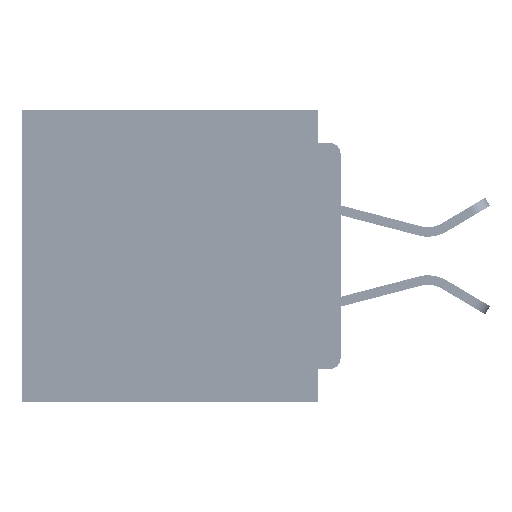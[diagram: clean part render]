
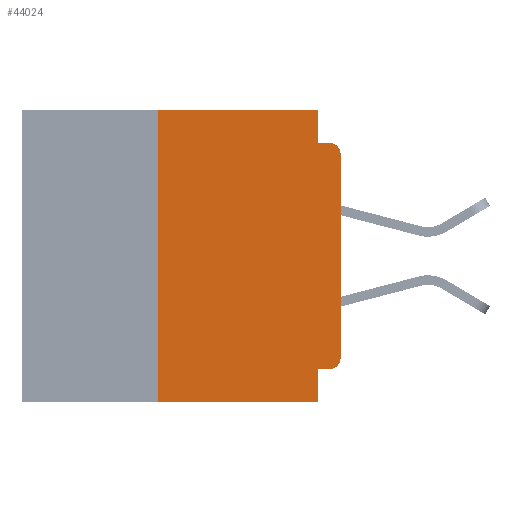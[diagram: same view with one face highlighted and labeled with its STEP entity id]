
A CAD part, left-side view. The second image highlights one B-rep face of the part: STEP entity #44024.
In plain terms, the highlighted planar face has unit normal (-1, 0, 0).
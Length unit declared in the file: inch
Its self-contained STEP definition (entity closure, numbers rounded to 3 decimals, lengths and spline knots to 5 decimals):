
#98 = DIRECTION ( 'NONE',  ( 1., 0., 0. ) ) ;
#563 = CARTESIAN_POINT ( 'NONE',  ( 0., 0.437, 0. ) ) ;
#869 = CIRCLE ( 'NONE', #25899, 0.015 ) ;
#2628 = VERTEX_POINT ( 'NONE', #38339 ) ;
#2960 = DIRECTION ( 'NONE',  ( -1., 0., 0. ) ) ;
#3124 = CIRCLE ( 'NONE', #36083, 0.015 ) ;
#3343 = EDGE_LOOP ( 'NONE', ( #52701, #41133, #58775, #60314, #26723, #52760, #15186, #45871, #8258, #12189 ) ) ;
#4657 = VERTEX_POINT ( 'NONE', #30805 ) ;
#6413 = VECTOR ( 'NONE', #18848, 39.37008 ) ;
#7046 = CARTESIAN_POINT ( 'NONE',  ( 0., 0.031, 0. ) ) ;
#7958 = LINE ( 'NONE', #43260, #6413 ) ;
#8258 = ORIENTED_EDGE ( 'NONE', *, *, #57988, .F. ) ;
#8402 = DIRECTION ( 'NONE',  ( 0., 1., 0. ) ) ;
#9303 = VERTEX_POINT ( 'NONE', #39330 ) ;
#12189 = ORIENTED_EDGE ( 'NONE', *, *, #32859, .T. ) ;
#14083 = LINE ( 'NONE', #53058, #51657 ) ;
#15186 = ORIENTED_EDGE ( 'NONE', *, *, #61107, .T. ) ;
#17028 = LINE ( 'NONE', #18074, #39983 ) ;
#18074 = CARTESIAN_POINT ( 'NONE',  ( 0., 0., -0.355 ) ) ;
#18848 = DIRECTION ( 'NONE',  ( 0., 0., -1. ) ) ;
#20015 = CARTESIAN_POINT ( 'NONE',  ( 0., 0.015, -0.355 ) ) ;
#20084 = CARTESIAN_POINT ( 'NONE',  ( 0., 0.437, -0.4 ) ) ;
#20939 = CARTESIAN_POINT ( 'NONE',  ( 0., 0.25, -0.4 ) ) ;
#21856 = LINE ( 'NONE', #30846, #47942 ) ;
#22065 = EDGE_CURVE ( 'NONE', #60674, #9303, #14083, .T. ) ;
#22498 = DIRECTION ( 'NONE',  ( 0., -1., 0. ) ) ;
#23489 = EDGE_CURVE ( 'NONE', #28039, #43343, #21856, .T. ) ;
#23637 = LINE ( 'NONE', #20084, #48149 ) ;
#24789 = CARTESIAN_POINT ( 'NONE',  ( 0., 0., -0.06 ) ) ;
#25058 = DIRECTION ( 'NONE',  ( 0., -1., 0. ) ) ;
#25899 = AXIS2_PLACEMENT_3D ( 'NONE', #56039, #26727, #60895 ) ;
#26045 = VECTOR ( 'NONE', #35021, 39.37008 ) ;
#26723 = ORIENTED_EDGE ( 'NONE', *, *, #46386, .F. ) ;
#26727 = DIRECTION ( 'NONE',  ( -1., 0., 0. ) ) ;
#28039 = VERTEX_POINT ( 'NONE', #62987 ) ;
#28452 = DIRECTION ( 'NONE',  ( 0., 0., -1. ) ) ;
#29638 = PLANE ( 'NONE',  #37920 ) ;
#30805 = CARTESIAN_POINT ( 'NONE',  ( 0., 0.015, -0.045 ) ) ;
#30846 = CARTESIAN_POINT ( 'NONE',  ( 0., 0., 0. ) ) ;
#31101 = CARTESIAN_POINT ( 'NONE',  ( 0., 0.25, -0.4 ) ) ;
#32452 = CARTESIAN_POINT ( 'NONE',  ( 0., 0.015, -0.34 ) ) ;
#32859 = EDGE_CURVE ( 'NONE', #36303, #28039, #3124, .T. ) ;
#34471 = CARTESIAN_POINT ( 'NONE',  ( 0., 0.031, -0.4 ) ) ;
#34568 = DIRECTION ( 'NONE',  ( 0., 0., -1. ) ) ;
#35021 = DIRECTION ( 'NONE',  ( 0., -1., 0. ) ) ;
#35789 = EDGE_CURVE ( 'NONE', #41170, #2628, #40969, .T. ) ;
#35803 = VECTOR ( 'NONE', #22498, 39.37008 ) ;
#36083 = AXIS2_PLACEMENT_3D ( 'NONE', #32452, #2960, #37370 ) ;
#36303 = VERTEX_POINT ( 'NONE', #20015 ) ;
#37370 = DIRECTION ( 'NONE',  ( 0., 0., -1. ) ) ;
#37485 = LINE ( 'NONE', #563, #26045 ) ;
#37920 = AXIS2_PLACEMENT_3D ( 'NONE', #44146, #98, #34568 ) ;
#38339 = CARTESIAN_POINT ( 'NONE',  ( 0., 0.25, 0. ) ) ;
#38690 = VERTEX_POINT ( 'NONE', #41377 ) ;
#38811 = LINE ( 'NONE', #61409, #35803 ) ;
#39330 = CARTESIAN_POINT ( 'NONE',  ( 0., 0.031, -0.045 ) ) ;
#39983 = VECTOR ( 'NONE', #8402, 39.37008 ) ;
#40969 = LINE ( 'NONE', #20939, #52534 ) ;
#41133 = ORIENTED_EDGE ( 'NONE', *, *, #48508, .T. ) ;
#41170 = VERTEX_POINT ( 'NONE', #31101 ) ;
#41377 = CARTESIAN_POINT ( 'NONE',  ( 0., 0.031, -0.355 ) ) ;
#43260 = CARTESIAN_POINT ( 'NONE',  ( 0., 0.031, -0.4 ) ) ;
#43343 = VERTEX_POINT ( 'NONE', #24789 ) ;
#43917 = FACE_OUTER_BOUND ( 'NONE', #3343, .T. ) ;
#44024 = ADVANCED_FACE ( 'NONE', ( #43917 ), #29638, .F. ) ;
#44146 = CARTESIAN_POINT ( 'NONE',  ( 0., 0.437, 0. ) ) ;
#45871 = ORIENTED_EDGE ( 'NONE', *, *, #56843, .F. ) ;
#46386 = EDGE_CURVE ( 'NONE', #2628, #60674, #37485, .T. ) ;
#47942 = VECTOR ( 'NONE', #60102, 39.37008 ) ;
#48149 = VECTOR ( 'NONE', #25058, 39.37008 ) ;
#48508 = EDGE_CURVE ( 'NONE', #43343, #4657, #869, .T. ) ;
#50531 = DIRECTION ( 'NONE',  ( 0., 0., 1. ) ) ;
#51657 = VECTOR ( 'NONE', #28452, 39.37008 ) ;
#52534 = VECTOR ( 'NONE', #50531, 39.37008 ) ;
#52701 = ORIENTED_EDGE ( 'NONE', *, *, #23489, .T. ) ;
#52760 = ORIENTED_EDGE ( 'NONE', *, *, #35789, .F. ) ;
#53058 = CARTESIAN_POINT ( 'NONE',  ( 0., 0.031, 0. ) ) ;
#54794 = EDGE_CURVE ( 'NONE', #9303, #4657, #38811, .T. ) ;
#55101 = VERTEX_POINT ( 'NONE', #34471 ) ;
#56039 = CARTESIAN_POINT ( 'NONE',  ( 0., 0.015, -0.06 ) ) ;
#56843 = EDGE_CURVE ( 'NONE', #38690, #55101, #7958, .T. ) ;
#57988 = EDGE_CURVE ( 'NONE', #36303, #38690, #17028, .T. ) ;
#58775 = ORIENTED_EDGE ( 'NONE', *, *, #54794, .F. ) ;
#60102 = DIRECTION ( 'NONE',  ( 0., 0., 1. ) ) ;
#60314 = ORIENTED_EDGE ( 'NONE', *, *, #22065, .F. ) ;
#60674 = VERTEX_POINT ( 'NONE', #7046 ) ;
#60895 = DIRECTION ( 'NONE',  ( 0., 0., -1. ) ) ;
#61107 = EDGE_CURVE ( 'NONE', #41170, #55101, #23637, .T. ) ;
#61409 = CARTESIAN_POINT ( 'NONE',  ( 0., 0., -0.045 ) ) ;
#62987 = CARTESIAN_POINT ( 'NONE',  ( 0., 0., -0.34 ) ) ;
